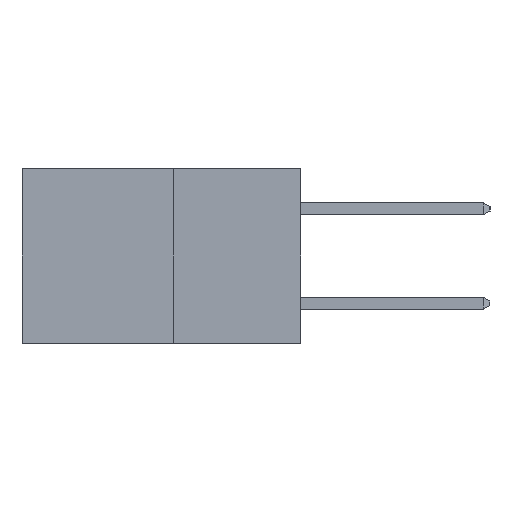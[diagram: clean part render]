
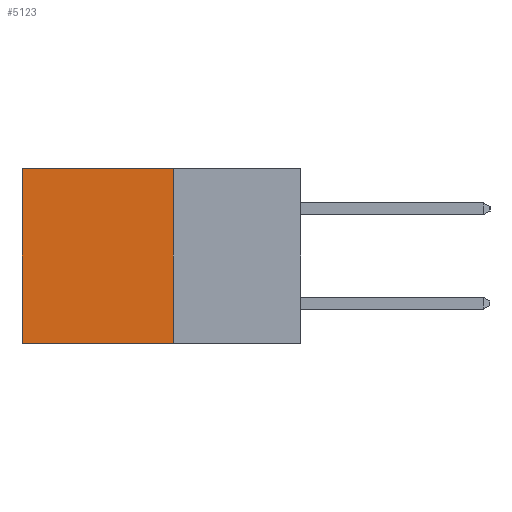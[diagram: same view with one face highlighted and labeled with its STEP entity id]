
A CAD part, left-side view. The second image highlights one B-rep face of the part: STEP entity #5123.
In plain terms, the highlighted planar face has unit normal (-1, 0, 0).
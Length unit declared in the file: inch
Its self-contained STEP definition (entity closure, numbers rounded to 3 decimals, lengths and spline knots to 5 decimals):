
#514 = VECTOR ( 'NONE', #3191, 39.37008 ) ;
#1253 = CARTESIAN_POINT ( 'NONE',  ( 0.277, 0.27, 0. ) ) ;
#1458 = EDGE_CURVE ( 'NONE', #5637, #7421, #9181, .T. ) ;
#2258 = CARTESIAN_POINT ( 'NONE',  ( 0.277, 0.27, -0.37 ) ) ;
#2416 = DIRECTION ( 'NONE',  ( 0., 1., 0. ) ) ;
#2734 = CARTESIAN_POINT ( 'NONE',  ( 0.277, 0.27, 0. ) ) ;
#2814 = CARTESIAN_POINT ( 'NONE',  ( 0.277, 0.27, -0.37 ) ) ;
#3000 = VECTOR ( 'NONE', #2416, 39.37008 ) ;
#3077 = CARTESIAN_POINT ( 'NONE',  ( 0.277, 0.27, -0.37 ) ) ;
#3191 = DIRECTION ( 'NONE',  ( 0., 0., -1. ) ) ;
#3239 = DIRECTION ( 'NONE',  ( 0., 0., -1. ) ) ;
#3251 = DIRECTION ( 'NONE',  ( 1., 0., 0. ) ) ;
#3442 = CARTESIAN_POINT ( 'NONE',  ( 0.277, 0.27, -0.37 ) ) ;
#3619 = LINE ( 'NONE', #2258, #514 ) ;
#3647 = PLANE ( 'NONE',  #6490 ) ;
#3787 = CARTESIAN_POINT ( 'NONE',  ( 0.277, 0.59, 0. ) ) ;
#4196 = EDGE_CURVE ( 'NONE', #7074, #5575, #5412, .T. ) ;
#4469 = ORIENTED_EDGE ( 'NONE', *, *, #4196, .T. ) ;
#4478 = VECTOR ( 'NONE', #10853, 39.37008 ) ;
#4714 = VECTOR ( 'NONE', #8818, 39.37008 ) ;
#5123 = ADVANCED_FACE ( 'NONE', ( #9245 ), #3647, .F. ) ;
#5154 = ORIENTED_EDGE ( 'NONE', *, *, #11354, .T. ) ;
#5412 = LINE ( 'NONE', #2734, #3000 ) ;
#5575 = VERTEX_POINT ( 'NONE', #3787 ) ;
#5637 = VERTEX_POINT ( 'NONE', #3077 ) ;
#6490 = AXIS2_PLACEMENT_3D ( 'NONE', #3442, #3251, #3239 ) ;
#6804 = LINE ( 'NONE', #9708, #4714 ) ;
#7022 = ORIENTED_EDGE ( 'NONE', *, *, #9046, .F. ) ;
#7074 = VERTEX_POINT ( 'NONE', #1253 ) ;
#7421 = VERTEX_POINT ( 'NONE', #9729 ) ;
#8818 = DIRECTION ( 'NONE',  ( 0., 0., -1. ) ) ;
#9046 = EDGE_CURVE ( 'NONE', #7074, #5637, #3619, .T. ) ;
#9181 = LINE ( 'NONE', #2814, #4478 ) ;
#9245 = FACE_OUTER_BOUND ( 'NONE', #9718, .T. ) ;
#9708 = CARTESIAN_POINT ( 'NONE',  ( 0.277, 0.59, -0.37 ) ) ;
#9718 = EDGE_LOOP ( 'NONE', ( #5154, #10129, #7022, #4469 ) ) ;
#9729 = CARTESIAN_POINT ( 'NONE',  ( 0.277, 0.59, -0.37 ) ) ;
#10129 = ORIENTED_EDGE ( 'NONE', *, *, #1458, .F. ) ;
#10853 = DIRECTION ( 'NONE',  ( 0., 1., 0. ) ) ;
#11354 = EDGE_CURVE ( 'NONE', #5575, #7421, #6804, .T. ) ;
